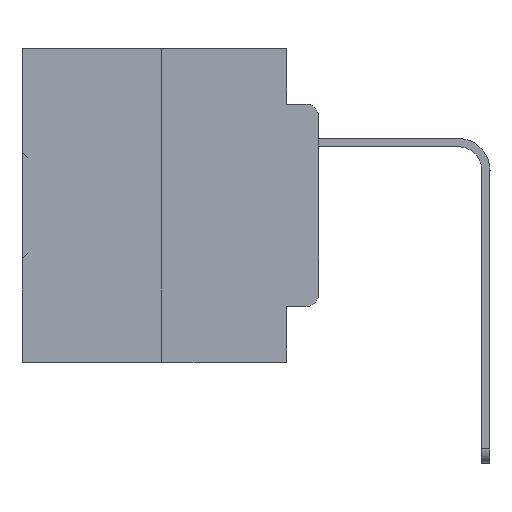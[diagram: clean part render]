
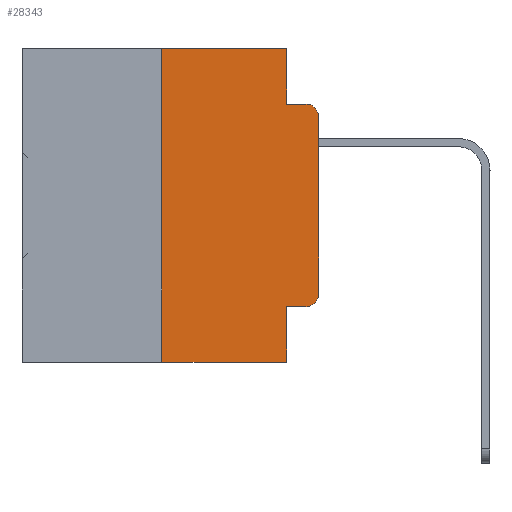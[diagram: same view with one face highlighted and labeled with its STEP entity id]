
A CAD part, left-side view. The second image highlights one B-rep face of the part: STEP entity #28343.
In plain terms, the highlighted planar face has unit normal (-1, 0, 0).
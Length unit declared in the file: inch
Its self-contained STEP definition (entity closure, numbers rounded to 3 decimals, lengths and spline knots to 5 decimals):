
#933 = FACE_OUTER_BOUND ( 'NONE', #32669, .T. ) ;
#2452 = DIRECTION ( 'NONE',  ( 0., 0., 1. ) ) ;
#3855 = ORIENTED_EDGE ( 'NONE', *, *, #6452, .F. ) ;
#4105 = LINE ( 'NONE', #21052, #23552 ) ;
#4242 = EDGE_CURVE ( 'NONE', #29157, #23795, #29474, .T. ) ;
#4718 = VERTEX_POINT ( 'NONE', #24152 ) ;
#5196 = DIRECTION ( 'NONE',  ( 0., -1., 0. ) ) ;
#5551 = DIRECTION ( 'NONE',  ( 0., -1., 0. ) ) ;
#6239 = VECTOR ( 'NONE', #18134, 39.37008 ) ;
#6359 = VERTEX_POINT ( 'NONE', #10001 ) ;
#6452 = EDGE_CURVE ( 'NONE', #29092, #4718, #30929, .T. ) ;
#6534 = VERTEX_POINT ( 'NONE', #13411 ) ;
#7051 = CARTESIAN_POINT ( 'NONE',  ( 0., 0.02, -0.1085 ) ) ;
#7933 = CARTESIAN_POINT ( 'NONE',  ( 0., 0.473, 0. ) ) ;
#8302 = CARTESIAN_POINT ( 'NONE',  ( 0., 0.051, 0. ) ) ;
#8653 = DIRECTION ( 'NONE',  ( 0., 0., -1. ) ) ;
#9888 = CARTESIAN_POINT ( 'NONE',  ( 0., 0., 0. ) ) ;
#10001 = CARTESIAN_POINT ( 'NONE',  ( 0., 0., -0.3915 ) ) ;
#10044 = DIRECTION ( 'NONE',  ( 0., 0., -1. ) ) ;
#10386 = AXIS2_PLACEMENT_3D ( 'NONE', #15528, #21118, #24009 ) ;
#10538 = AXIS2_PLACEMENT_3D ( 'NONE', #19456, #33478, #8653 ) ;
#11885 = LINE ( 'NONE', #8302, #34820 ) ;
#12167 = LINE ( 'NONE', #24906, #23412 ) ;
#12188 = CARTESIAN_POINT ( 'NONE',  ( 0., 0.051, -0.4115 ) ) ;
#12193 = EDGE_CURVE ( 'NONE', #24665, #27949, #15002, .T. ) ;
#13305 = DIRECTION ( 'NONE',  ( 0., 0., -1. ) ) ;
#13411 = CARTESIAN_POINT ( 'NONE',  ( 0., 0., -0.1085 ) ) ;
#13430 = CARTESIAN_POINT ( 'NONE',  ( 0., 0.051, -0.0885 ) ) ;
#14006 = EDGE_CURVE ( 'NONE', #6359, #6534, #30043, .T. ) ;
#14262 = ORIENTED_EDGE ( 'NONE', *, *, #30019, .F. ) ;
#15002 = LINE ( 'NONE', #24779, #30593 ) ;
#15528 = CARTESIAN_POINT ( 'NONE',  ( 0., 0.473, 0. ) ) ;
#15892 = CARTESIAN_POINT ( 'NONE',  ( 0., 0.02, -0.4115 ) ) ;
#15916 = EDGE_CURVE ( 'NONE', #25464, #6359, #31228, .T. ) ;
#16536 = CARTESIAN_POINT ( 'NONE',  ( 0., 0.25, -0.5 ) ) ;
#16783 = DIRECTION ( 'NONE',  ( 0., -1., 0. ) ) ;
#16896 = VECTOR ( 'NONE', #5551, 39.37008 ) ;
#17272 = ORIENTED_EDGE ( 'NONE', *, *, #22967, .F. ) ;
#18134 = DIRECTION ( 'NONE',  ( 0., 0., 1. ) ) ;
#18313 = EDGE_CURVE ( 'NONE', #6534, #23795, #32384, .T. ) ;
#18793 = ORIENTED_EDGE ( 'NONE', *, *, #21544, .T. ) ;
#19456 = CARTESIAN_POINT ( 'NONE',  ( 0., 0.02, -0.3915 ) ) ;
#20218 = ORIENTED_EDGE ( 'NONE', *, *, #4242, .F. ) ;
#21052 = CARTESIAN_POINT ( 'NONE',  ( 0., 0.051, -0.4115 ) ) ;
#21118 = DIRECTION ( 'NONE',  ( 1., 0., 0. ) ) ;
#21544 = EDGE_CURVE ( 'NONE', #24665, #25464, #4105, .T. ) ;
#22967 = EDGE_CURVE ( 'NONE', #34551, #29092, #12167, .T. ) ;
#23412 = VECTOR ( 'NONE', #2452, 39.37008 ) ;
#23552 = VECTOR ( 'NONE', #29249, 39.37008 ) ;
#23795 = VERTEX_POINT ( 'NONE', #28731 ) ;
#23865 = ORIENTED_EDGE ( 'NONE', *, *, #18313, .T. ) ;
#24009 = DIRECTION ( 'NONE',  ( 0., 0., -1. ) ) ;
#24016 = VECTOR ( 'NONE', #5196, 39.37008 ) ;
#24095 = AXIS2_PLACEMENT_3D ( 'NONE', #7051, #34836, #10044 ) ;
#24152 = CARTESIAN_POINT ( 'NONE',  ( 0., 0.051, 0. ) ) ;
#24665 = VERTEX_POINT ( 'NONE', #12188 ) ;
#24666 = CARTESIAN_POINT ( 'NONE',  ( 0., 0.473, -0.5 ) ) ;
#24779 = CARTESIAN_POINT ( 'NONE',  ( 0., 0.051, 0. ) ) ;
#24906 = CARTESIAN_POINT ( 'NONE',  ( 0., 0.25, 0. ) ) ;
#25253 = CARTESIAN_POINT ( 'NONE',  ( 0., 0.051, -0.0885 ) ) ;
#25464 = VERTEX_POINT ( 'NONE', #15892 ) ;
#26250 = EDGE_CURVE ( 'NONE', #34551, #27949, #31825, .T. ) ;
#26281 = PLANE ( 'NONE',  #10386 ) ;
#27688 = DIRECTION ( 'NONE',  ( 0., 0., -1. ) ) ;
#27764 = CARTESIAN_POINT ( 'NONE',  ( 0., 0.051, -0.5 ) ) ;
#27924 = ORIENTED_EDGE ( 'NONE', *, *, #12193, .F. ) ;
#27949 = VERTEX_POINT ( 'NONE', #27764 ) ;
#28343 = ADVANCED_FACE ( 'NONE', ( #933 ), #26281, .F. ) ;
#28731 = CARTESIAN_POINT ( 'NONE',  ( 0., 0.02, -0.0885 ) ) ;
#29092 = VERTEX_POINT ( 'NONE', #32758 ) ;
#29157 = VERTEX_POINT ( 'NONE', #13430 ) ;
#29249 = DIRECTION ( 'NONE',  ( 0., -1., 0. ) ) ;
#29474 = LINE ( 'NONE', #25253, #16896 ) ;
#30019 = EDGE_CURVE ( 'NONE', #4718, #29157, #11885, .T. ) ;
#30043 = LINE ( 'NONE', #9888, #6239 ) ;
#30092 = VECTOR ( 'NONE', #16783, 39.37008 ) ;
#30593 = VECTOR ( 'NONE', #13305, 39.37008 ) ;
#30929 = LINE ( 'NONE', #7933, #24016 ) ;
#31228 = CIRCLE ( 'NONE', #10538, 0.02 ) ;
#31825 = LINE ( 'NONE', #24666, #30092 ) ;
#32254 = ORIENTED_EDGE ( 'NONE', *, *, #14006, .T. ) ;
#32384 = CIRCLE ( 'NONE', #24095, 0.02 ) ;
#32669 = EDGE_LOOP ( 'NONE', ( #32254, #23865, #20218, #14262, #3855, #17272, #33665, #27924, #18793, #33779 ) ) ;
#32758 = CARTESIAN_POINT ( 'NONE',  ( 0., 0.25, 0. ) ) ;
#33478 = DIRECTION ( 'NONE',  ( -1., 0., 0. ) ) ;
#33665 = ORIENTED_EDGE ( 'NONE', *, *, #26250, .T. ) ;
#33779 = ORIENTED_EDGE ( 'NONE', *, *, #15916, .T. ) ;
#34551 = VERTEX_POINT ( 'NONE', #16536 ) ;
#34820 = VECTOR ( 'NONE', #27688, 39.37008 ) ;
#34836 = DIRECTION ( 'NONE',  ( -1., 0., 0. ) ) ;
